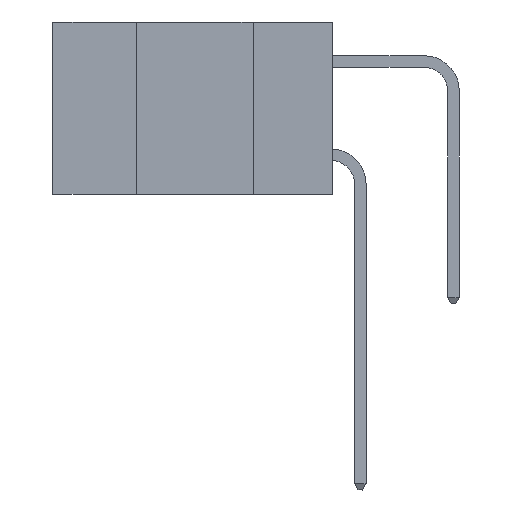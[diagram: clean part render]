
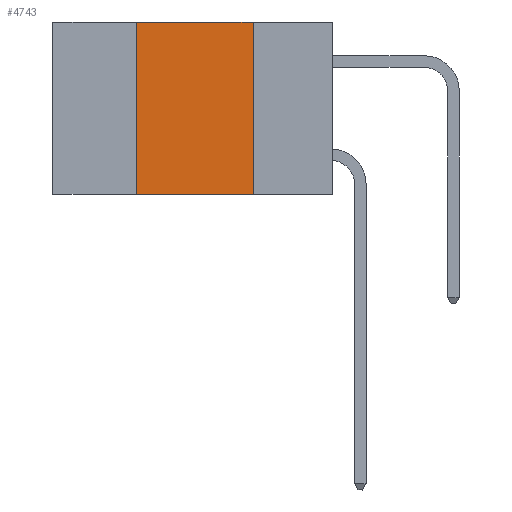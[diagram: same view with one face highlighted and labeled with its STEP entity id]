
A CAD part, left-side view. The second image highlights one B-rep face of the part: STEP entity #4743.
In plain terms, the highlighted planar face has unit normal (-1, 0, 0).
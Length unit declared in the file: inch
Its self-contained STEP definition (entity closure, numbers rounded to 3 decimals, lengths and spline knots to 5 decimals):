
#32 = DIRECTION ( 'NONE',  ( 0., -1., 0. ) ) ;
#719 = ORIENTED_EDGE ( 'NONE', *, *, #12703, .T. ) ;
#1617 = CARTESIAN_POINT ( 'NONE',  ( 0., 0.42, 0. ) ) ;
#1721 = VERTEX_POINT ( 'NONE', #13684 ) ;
#1992 = EDGE_CURVE ( 'NONE', #18194, #1721, #11910, .T. ) ;
#2228 = VERTEX_POINT ( 'NONE', #4803 ) ;
#3381 = DIRECTION ( 'NONE',  ( 0., 0., -1. ) ) ;
#3543 = LINE ( 'NONE', #10655, #9501 ) ;
#3834 = EDGE_CURVE ( 'NONE', #10636, #18194, #7696, .T. ) ;
#4743 = ADVANCED_FACE ( 'NONE', ( #18661 ), #16837, .F. ) ;
#4803 = CARTESIAN_POINT ( 'NONE',  ( 0., 0.17, -0.37 ) ) ;
#5670 = ORIENTED_EDGE ( 'NONE', *, *, #1992, .F. ) ;
#5824 = EDGE_CURVE ( 'NONE', #1721, #2228, #3543, .T. ) ;
#6069 = CARTESIAN_POINT ( 'NONE',  ( 0., 0.6, -0.37 ) ) ;
#6462 = CARTESIAN_POINT ( 'NONE',  ( 0., 0.6, 0. ) ) ;
#6616 = ORIENTED_EDGE ( 'NONE', *, *, #3834, .F. ) ;
#6999 = VECTOR ( 'NONE', #32, 39.37008 ) ;
#7180 = DIRECTION ( 'NONE',  ( 0., 0., 1. ) ) ;
#7309 = CARTESIAN_POINT ( 'NONE',  ( 0., 0.42, 0. ) ) ;
#7696 = LINE ( 'NONE', #7309, #13839 ) ;
#8054 = VECTOR ( 'NONE', #16014, 39.37008 ) ;
#9483 = DIRECTION ( 'NONE',  ( 1., 0., 0. ) ) ;
#9501 = VECTOR ( 'NONE', #3381, 39.37008 ) ;
#10636 = VERTEX_POINT ( 'NONE', #12084 ) ;
#10655 = CARTESIAN_POINT ( 'NONE',  ( 0., 0.17, 0. ) ) ;
#10663 = EDGE_LOOP ( 'NONE', ( #18491, #5670, #6616, #719 ) ) ;
#11910 = LINE ( 'NONE', #16276, #8054 ) ;
#12084 = CARTESIAN_POINT ( 'NONE',  ( 0., 0.42, -0.37 ) ) ;
#12296 = AXIS2_PLACEMENT_3D ( 'NONE', #6462, #9483, #16784 ) ;
#12299 = LINE ( 'NONE', #6069, #6999 ) ;
#12703 = EDGE_CURVE ( 'NONE', #10636, #2228, #12299, .T. ) ;
#13684 = CARTESIAN_POINT ( 'NONE',  ( 0., 0.17, 0. ) ) ;
#13839 = VECTOR ( 'NONE', #7180, 39.37008 ) ;
#16014 = DIRECTION ( 'NONE',  ( 0., -1., 0. ) ) ;
#16276 = CARTESIAN_POINT ( 'NONE',  ( 0., 0.6, 0. ) ) ;
#16784 = DIRECTION ( 'NONE',  ( 0., 0., -1. ) ) ;
#16837 = PLANE ( 'NONE',  #12296 ) ;
#18194 = VERTEX_POINT ( 'NONE', #1617 ) ;
#18491 = ORIENTED_EDGE ( 'NONE', *, *, #5824, .F. ) ;
#18661 = FACE_OUTER_BOUND ( 'NONE', #10663, .T. ) ;
